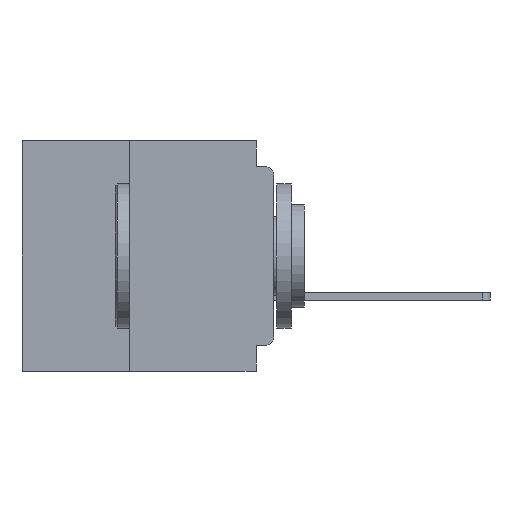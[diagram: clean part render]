
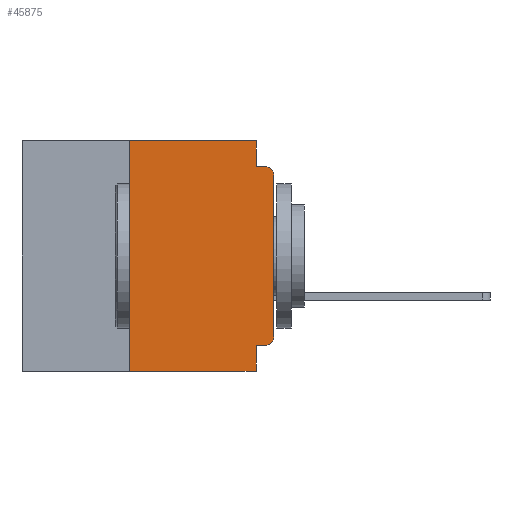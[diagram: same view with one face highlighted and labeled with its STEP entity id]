
A CAD part, left-side view. The second image highlights one B-rep face of the part: STEP entity #45875.
In plain terms, the highlighted planar face has unit normal (-1, 0, 0).
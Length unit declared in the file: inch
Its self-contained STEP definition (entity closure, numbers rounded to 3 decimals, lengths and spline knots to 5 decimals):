
#402 = CARTESIAN_POINT ( 'NONE',  ( 0., 0.437, 0. ) ) ;
#946 = EDGE_CURVE ( 'NONE', #11784, #28207, #57535, .T. ) ;
#1026 = CARTESIAN_POINT ( 'NONE',  ( 0., 0., 0. ) ) ;
#1418 = VERTEX_POINT ( 'NONE', #9619 ) ;
#1844 = EDGE_LOOP ( 'NONE', ( #27337, #27686, #8515, #28583, #17949, #64518, #42675, #40331, #24850, #27814 ) ) ;
#4230 = FACE_OUTER_BOUND ( 'NONE', #1844, .T. ) ;
#5359 = VECTOR ( 'NONE', #28954, 39.37008 ) ;
#5473 = CARTESIAN_POINT ( 'NONE',  ( 0., 0.437, -0.4 ) ) ;
#7569 = LINE ( 'NONE', #40668, #34934 ) ;
#8370 = CARTESIAN_POINT ( 'NONE',  ( 0., 0., -0.34 ) ) ;
#8515 = ORIENTED_EDGE ( 'NONE', *, *, #22812, .F. ) ;
#9309 = CARTESIAN_POINT ( 'NONE',  ( 0., 0., -0.06 ) ) ;
#9485 = DIRECTION ( 'NONE',  ( 0., 0., -1. ) ) ;
#9619 = CARTESIAN_POINT ( 'NONE',  ( 0., 0.25, -0.4 ) ) ;
#10020 = DIRECTION ( 'NONE',  ( 0., -1., 0. ) ) ;
#10757 = LINE ( 'NONE', #36675, #36442 ) ;
#11511 = VECTOR ( 'NONE', #23089, 39.37008 ) ;
#11784 = VERTEX_POINT ( 'NONE', #9309 ) ;
#12206 = DIRECTION ( 'NONE',  ( -1., 0., 0. ) ) ;
#12898 = LINE ( 'NONE', #64816, #26700 ) ;
#13146 = VERTEX_POINT ( 'NONE', #8370 ) ;
#13155 = EDGE_CURVE ( 'NONE', #53411, #55227, #12898, .T. ) ;
#13473 = LINE ( 'NONE', #5473, #66114 ) ;
#16233 = CARTESIAN_POINT ( 'NONE',  ( 0., 0.015, -0.045 ) ) ;
#17949 = ORIENTED_EDGE ( 'NONE', *, *, #55179, .F. ) ;
#18585 = CARTESIAN_POINT ( 'NONE',  ( 0., 0.031, -0.4 ) ) ;
#19747 = AXIS2_PLACEMENT_3D ( 'NONE', #402, #56692, #26374 ) ;
#19914 = CARTESIAN_POINT ( 'NONE',  ( 0., 0.031, 0. ) ) ;
#20873 = VECTOR ( 'NONE', #9485, 39.37008 ) ;
#21408 = VERTEX_POINT ( 'NONE', #60328 ) ;
#22621 = EDGE_CURVE ( 'NONE', #1418, #47103, #10757, .T. ) ;
#22812 = EDGE_CURVE ( 'NONE', #21408, #28207, #65777, .T. ) ;
#23066 = AXIS2_PLACEMENT_3D ( 'NONE', #42828, #12206, #47934 ) ;
#23089 = DIRECTION ( 'NONE',  ( 0., -1., 0. ) ) ;
#24850 = ORIENTED_EDGE ( 'NONE', *, *, #13155, .F. ) ;
#25433 = CARTESIAN_POINT ( 'NONE',  ( 0., 0.031, -0.4 ) ) ;
#26374 = DIRECTION ( 'NONE',  ( 0., 0., -1. ) ) ;
#26700 = VECTOR ( 'NONE', #29386, 39.37008 ) ;
#27084 = VERTEX_POINT ( 'NONE', #47581 ) ;
#27337 = ORIENTED_EDGE ( 'NONE', *, *, #50481, .T. ) ;
#27686 = ORIENTED_EDGE ( 'NONE', *, *, #946, .T. ) ;
#27814 = ORIENTED_EDGE ( 'NONE', *, *, #65101, .T. ) ;
#28207 = VERTEX_POINT ( 'NONE', #16233 ) ;
#28583 = ORIENTED_EDGE ( 'NONE', *, *, #48355, .F. ) ;
#28954 = DIRECTION ( 'NONE',  ( 0., 0., -1. ) ) ;
#29386 = DIRECTION ( 'NONE',  ( 0., 1., 0. ) ) ;
#30775 = CARTESIAN_POINT ( 'NONE',  ( 0., 0.031, -0.355 ) ) ;
#31379 = CIRCLE ( 'NONE', #23066, 0.015 ) ;
#32756 = LINE ( 'NONE', #18585, #5359 ) ;
#34934 = VECTOR ( 'NONE', #10020, 39.37008 ) ;
#36442 = VECTOR ( 'NONE', #41741, 39.37008 ) ;
#36675 = CARTESIAN_POINT ( 'NONE',  ( 0., 0.25, -0.4 ) ) ;
#38148 = AXIS2_PLACEMENT_3D ( 'NONE', #49692, #49643, #49628 ) ;
#39693 = EDGE_CURVE ( 'NONE', #1418, #44529, #13473, .T. ) ;
#40331 = ORIENTED_EDGE ( 'NONE', *, *, #60721, .F. ) ;
#40668 = CARTESIAN_POINT ( 'NONE',  ( 0., 0.437, 0. ) ) ;
#41741 = DIRECTION ( 'NONE',  ( 0., 0., 1. ) ) ;
#42675 = ORIENTED_EDGE ( 'NONE', *, *, #39693, .T. ) ;
#42828 = CARTESIAN_POINT ( 'NONE',  ( 0., 0.015, -0.34 ) ) ;
#44529 = VERTEX_POINT ( 'NONE', #25433 ) ;
#45875 = ADVANCED_FACE ( 'NONE', ( #4230 ), #51558, .F. ) ;
#47103 = VERTEX_POINT ( 'NONE', #64266 ) ;
#47581 = CARTESIAN_POINT ( 'NONE',  ( 0., 0.031, 0. ) ) ;
#47934 = DIRECTION ( 'NONE',  ( 0., 0., -1. ) ) ;
#48355 = EDGE_CURVE ( 'NONE', #27084, #21408, #49423, .T. ) ;
#48359 = CARTESIAN_POINT ( 'NONE',  ( 0., 0., -0.045 ) ) ;
#49107 = VECTOR ( 'NONE', #57080, 39.37008 ) ;
#49423 = LINE ( 'NONE', #19914, #20873 ) ;
#49628 = DIRECTION ( 'NONE',  ( 0., 0., -1. ) ) ;
#49643 = DIRECTION ( 'NONE',  ( -1., 0., 0. ) ) ;
#49692 = CARTESIAN_POINT ( 'NONE',  ( 0., 0.015, -0.06 ) ) ;
#50481 = EDGE_CURVE ( 'NONE', #13146, #11784, #64253, .T. ) ;
#51558 = PLANE ( 'NONE',  #19747 ) ;
#53411 = VERTEX_POINT ( 'NONE', #60230 ) ;
#55179 = EDGE_CURVE ( 'NONE', #47103, #27084, #7569, .T. ) ;
#55227 = VERTEX_POINT ( 'NONE', #30775 ) ;
#56692 = DIRECTION ( 'NONE',  ( 1., 0., 0. ) ) ;
#57080 = DIRECTION ( 'NONE',  ( 0., 0., 1. ) ) ;
#57535 = CIRCLE ( 'NONE', #38148, 0.015 ) ;
#60230 = CARTESIAN_POINT ( 'NONE',  ( 0., 0.015, -0.355 ) ) ;
#60328 = CARTESIAN_POINT ( 'NONE',  ( 0., 0.031, -0.045 ) ) ;
#60721 = EDGE_CURVE ( 'NONE', #55227, #44529, #32756, .T. ) ;
#61526 = DIRECTION ( 'NONE',  ( 0., -1., 0. ) ) ;
#64253 = LINE ( 'NONE', #1026, #49107 ) ;
#64266 = CARTESIAN_POINT ( 'NONE',  ( 0., 0.25, 0. ) ) ;
#64518 = ORIENTED_EDGE ( 'NONE', *, *, #22621, .F. ) ;
#64816 = CARTESIAN_POINT ( 'NONE',  ( 0., 0., -0.355 ) ) ;
#65101 = EDGE_CURVE ( 'NONE', #53411, #13146, #31379, .T. ) ;
#65777 = LINE ( 'NONE', #48359, #11511 ) ;
#66114 = VECTOR ( 'NONE', #61526, 39.37008 ) ;
